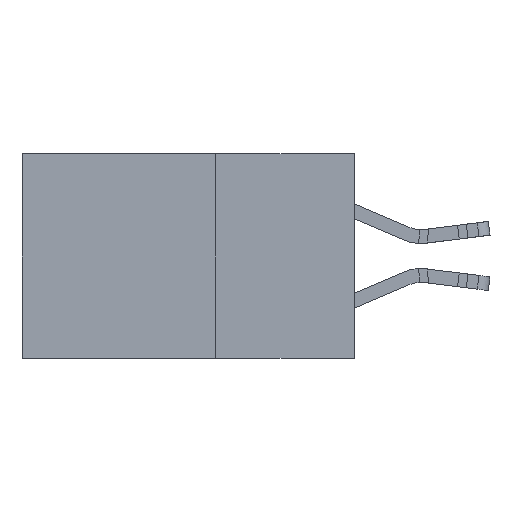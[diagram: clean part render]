
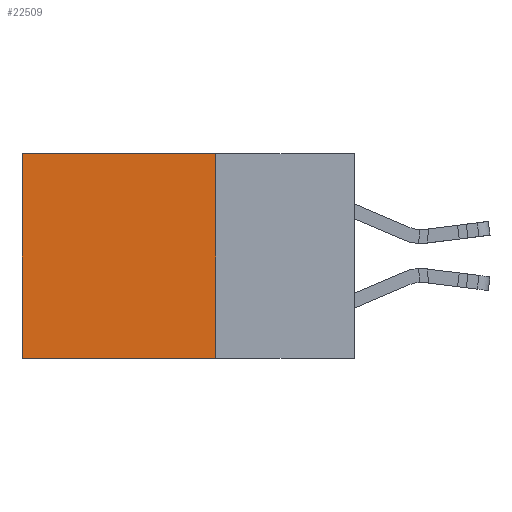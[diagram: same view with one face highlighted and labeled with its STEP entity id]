
A CAD part, left-side view. The second image highlights one B-rep face of the part: STEP entity #22509.
In plain terms, the highlighted planar face has unit normal (-1, 0, 0).
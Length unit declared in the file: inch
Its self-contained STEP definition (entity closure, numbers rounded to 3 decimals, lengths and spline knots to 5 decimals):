
#1774 = CARTESIAN_POINT ( 'NONE',  ( 0.2615, 0.25, 0. ) ) ;
#2202 = CARTESIAN_POINT ( 'NONE',  ( 0.2615, 0.6, -0.37 ) ) ;
#2295 = CARTESIAN_POINT ( 'NONE',  ( 0.2615, 0.25, -0.37 ) ) ;
#3863 = VERTEX_POINT ( 'NONE', #26750 ) ;
#4389 = LINE ( 'NONE', #25470, #23201 ) ;
#4794 = DIRECTION ( 'NONE',  ( 0., 0., -1. ) ) ;
#5334 = VECTOR ( 'NONE', #16967, 39.37008 ) ;
#5442 = EDGE_CURVE ( 'NONE', #15320, #3863, #14423, .T. ) ;
#5748 = CARTESIAN_POINT ( 'NONE',  ( 0.2615, 0.25, 0. ) ) ;
#7631 = VECTOR ( 'NONE', #10292, 39.37008 ) ;
#7850 = DIRECTION ( 'NONE',  ( 0., 1., 0. ) ) ;
#8302 = EDGE_CURVE ( 'NONE', #15320, #23117, #14633, .T. ) ;
#8496 = EDGE_CURVE ( 'NONE', #23117, #24938, #4389, .T. ) ;
#8630 = ORIENTED_EDGE ( 'NONE', *, *, #11631, .F. ) ;
#9666 = ORIENTED_EDGE ( 'NONE', *, *, #5442, .F. ) ;
#10292 = DIRECTION ( 'NONE',  ( 0., 0., -1. ) ) ;
#11631 = EDGE_CURVE ( 'NONE', #3863, #24938, #25717, .T. ) ;
#11778 = ORIENTED_EDGE ( 'NONE', *, *, #8302, .T. ) ;
#13866 = DIRECTION ( 'NONE',  ( 0., 0., -1. ) ) ;
#14376 = EDGE_LOOP ( 'NONE', ( #25041, #8630, #9666, #11778 ) ) ;
#14377 = CARTESIAN_POINT ( 'NONE',  ( 0.2615, 0.6, 0. ) ) ;
#14423 = LINE ( 'NONE', #27350, #7631 ) ;
#14633 = LINE ( 'NONE', #1774, #18280 ) ;
#15320 = VERTEX_POINT ( 'NONE', #5748 ) ;
#15792 = CARTESIAN_POINT ( 'NONE',  ( 0.2615, 0.25, -0.37 ) ) ;
#16967 = DIRECTION ( 'NONE',  ( 0., 1., 0. ) ) ;
#18280 = VECTOR ( 'NONE', #7850, 39.37008 ) ;
#22509 = ADVANCED_FACE ( 'NONE', ( #22740 ), #26359, .F. ) ;
#22740 = FACE_OUTER_BOUND ( 'NONE', #14376, .T. ) ;
#23117 = VERTEX_POINT ( 'NONE', #14377 ) ;
#23201 = VECTOR ( 'NONE', #4794, 39.37008 ) ;
#24693 = DIRECTION ( 'NONE',  ( 1., 0., 0. ) ) ;
#24938 = VERTEX_POINT ( 'NONE', #2202 ) ;
#25041 = ORIENTED_EDGE ( 'NONE', *, *, #8496, .T. ) ;
#25098 = AXIS2_PLACEMENT_3D ( 'NONE', #15792, #24693, #13866 ) ;
#25470 = CARTESIAN_POINT ( 'NONE',  ( 0.2615, 0.6, -0.37 ) ) ;
#25717 = LINE ( 'NONE', #2295, #5334 ) ;
#26359 = PLANE ( 'NONE',  #25098 ) ;
#26750 = CARTESIAN_POINT ( 'NONE',  ( 0.2615, 0.25, -0.37 ) ) ;
#27350 = CARTESIAN_POINT ( 'NONE',  ( 0.2615, 0.25, -0.37 ) ) ;
